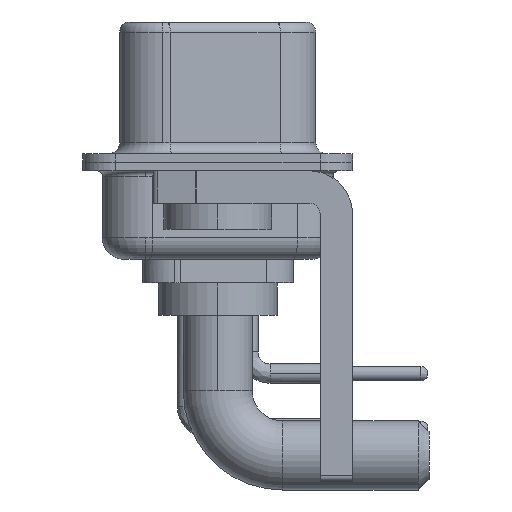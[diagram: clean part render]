
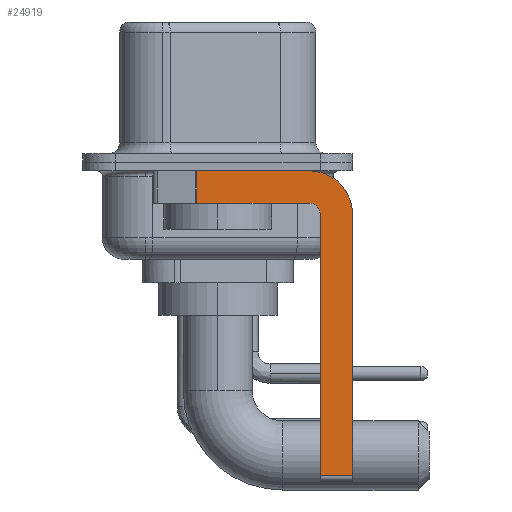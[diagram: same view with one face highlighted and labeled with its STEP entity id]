
A CAD part, left-side view. The second image highlights one B-rep face of the part: STEP entity #24919.
In plain terms, the highlighted planar face has unit normal (-1, 0, 0).
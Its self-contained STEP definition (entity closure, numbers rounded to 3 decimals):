
#395 = CARTESIAN_POINT ( 'NONE',  ( -2.9, 3., -0.4 ) ) ;
#840 = VECTOR ( 'NONE', #3299, 1000. ) ;
#975 = ORIENTED_EDGE ( 'NONE', *, *, #14896, .T. ) ;
#1237 = VECTOR ( 'NONE', #22251, 1000. ) ;
#1371 = CARTESIAN_POINT ( 'NONE',  ( -2.9, -4.25, -0.4 ) ) ;
#1502 = CARTESIAN_POINT ( 'NONE',  ( -2.9, -4.75, -14.55 ) ) ;
#3299 = DIRECTION ( 'NONE',  ( 0., 0., 1. ) ) ;
#3853 = VERTEX_POINT ( 'NONE', #1371 ) ;
#3903 = EDGE_CURVE ( 'NONE', #5203, #5998, #8963, .T. ) ;
#4202 = DIRECTION ( 'NONE',  ( 0., -1., 0. ) ) ;
#4449 = CARTESIAN_POINT ( 'NONE',  ( -2.9, -4.75, -2.4 ) ) ;
#4797 = DIRECTION ( 'NONE',  ( 0., 0., -1. ) ) ;
#4935 = ORIENTED_EDGE ( 'NONE', *, *, #19217, .F. ) ;
#5203 = VERTEX_POINT ( 'NONE', #1502 ) ;
#5998 = VERTEX_POINT ( 'NONE', #4449 ) ;
#7176 = CARTESIAN_POINT ( 'NONE',  ( -2.9, -4.25, -2.4 ) ) ;
#7457 = CARTESIAN_POINT ( 'NONE',  ( -2.9, 0.978, -1.9 ) ) ;
#7492 = ORIENTED_EDGE ( 'NONE', *, *, #21345, .F. ) ;
#7525 = VERTEX_POINT ( 'NONE', #7833 ) ;
#7827 = ORIENTED_EDGE ( 'NONE', *, *, #25107, .F. ) ;
#7833 = CARTESIAN_POINT ( 'NONE',  ( -2.9, -6.25, -2.4 ) ) ;
#8561 = VECTOR ( 'NONE', #23544, 1000. ) ;
#8839 = VECTOR ( 'NONE', #25263, 1000. ) ;
#8863 = ORIENTED_EDGE ( 'NONE', *, *, #3903, .F. ) ;
#8963 = LINE ( 'NONE', #25067, #840 ) ;
#10049 = ORIENTED_EDGE ( 'NONE', *, *, #15209, .F. ) ;
#10344 = CARTESIAN_POINT ( 'NONE',  ( -2.9, -6.25, -14.55 ) ) ;
#10887 = AXIS2_PLACEMENT_3D ( 'NONE', #23856, #20366, #4797 ) ;
#10991 = EDGE_LOOP ( 'NONE', ( #19746, #975, #7827, #10049, #8863, #25276, #4935, #7492 ) ) ;
#11230 = CIRCLE ( 'NONE', #13717, 2. ) ;
#11423 = VERTEX_POINT ( 'NONE', #19944 ) ;
#11783 = LINE ( 'NONE', #21588, #20483 ) ;
#12375 = DIRECTION ( 'NONE',  ( 0., 0., -1. ) ) ;
#12575 = LINE ( 'NONE', #395, #1237 ) ;
#12790 = EDGE_CURVE ( 'NONE', #5203, #17543, #11783, .T. ) ;
#13080 = DIRECTION ( 'NONE',  ( -1., 0., 0. ) ) ;
#13371 = LINE ( 'NONE', #15693, #8561 ) ;
#13717 = AXIS2_PLACEMENT_3D ( 'NONE', #24381, #22195, #14332 ) ;
#13925 = CARTESIAN_POINT ( 'NONE',  ( -2.9, -6.25, -2.4 ) ) ;
#14332 = DIRECTION ( 'NONE',  ( 0., 0., -1. ) ) ;
#14896 = EDGE_CURVE ( 'NONE', #20885, #15974, #13371, .T. ) ;
#15209 = EDGE_CURVE ( 'NONE', #5998, #11423, #17207, .T. ) ;
#15463 = LINE ( 'NONE', #17383, #8839 ) ;
#15693 = CARTESIAN_POINT ( 'NONE',  ( -2.9, 0.978, -1.9 ) ) ;
#15974 = VERTEX_POINT ( 'NONE', #7457 ) ;
#16000 = PLANE ( 'NONE',  #10887 ) ;
#16154 = EDGE_CURVE ( 'NONE', #20885, #3853, #12575, .T. ) ;
#17207 = CIRCLE ( 'NONE', #19273, 0.5 ) ;
#17257 = CARTESIAN_POINT ( 'NONE',  ( -2.9, 0.978, -0.4 ) ) ;
#17383 = CARTESIAN_POINT ( 'NONE',  ( -2.9, -4.25, -1.9 ) ) ;
#17543 = VERTEX_POINT ( 'NONE', #10344 ) ;
#17922 = FACE_OUTER_BOUND ( 'NONE', #10991, .T. ) ;
#19217 = EDGE_CURVE ( 'NONE', #7525, #17543, #23978, .T. ) ;
#19273 = AXIS2_PLACEMENT_3D ( 'NONE', #7176, #13080, #20955 ) ;
#19746 = ORIENTED_EDGE ( 'NONE', *, *, #16154, .F. ) ;
#19944 = CARTESIAN_POINT ( 'NONE',  ( -2.9, -4.25, -1.9 ) ) ;
#20366 = DIRECTION ( 'NONE',  ( 1., 0., 0. ) ) ;
#20483 = VECTOR ( 'NONE', #4202, 1000. ) ;
#20885 = VERTEX_POINT ( 'NONE', #17257 ) ;
#20955 = DIRECTION ( 'NONE',  ( 0., 0., 1. ) ) ;
#21345 = EDGE_CURVE ( 'NONE', #3853, #7525, #11230, .T. ) ;
#21588 = CARTESIAN_POINT ( 'NONE',  ( -2.9, -4.25, -14.55 ) ) ;
#22195 = DIRECTION ( 'NONE',  ( 1., 0., 0. ) ) ;
#22251 = DIRECTION ( 'NONE',  ( 0., -1., 0. ) ) ;
#23544 = DIRECTION ( 'NONE',  ( 0., 0., -1. ) ) ;
#23856 = CARTESIAN_POINT ( 'NONE',  ( -2.9, -4.25, -2.4 ) ) ;
#23978 = LINE ( 'NONE', #13925, #24717 ) ;
#24381 = CARTESIAN_POINT ( 'NONE',  ( -2.9, -4.25, -2.4 ) ) ;
#24717 = VECTOR ( 'NONE', #12375, 1000. ) ;
#24919 = ADVANCED_FACE ( 'NONE', ( #17922 ), #16000, .F. ) ;
#25067 = CARTESIAN_POINT ( 'NONE',  ( -2.9, -4.75, -14.8 ) ) ;
#25107 = EDGE_CURVE ( 'NONE', #11423, #15974, #15463, .T. ) ;
#25263 = DIRECTION ( 'NONE',  ( 0., 1., 0. ) ) ;
#25276 = ORIENTED_EDGE ( 'NONE', *, *, #12790, .T. ) ;
